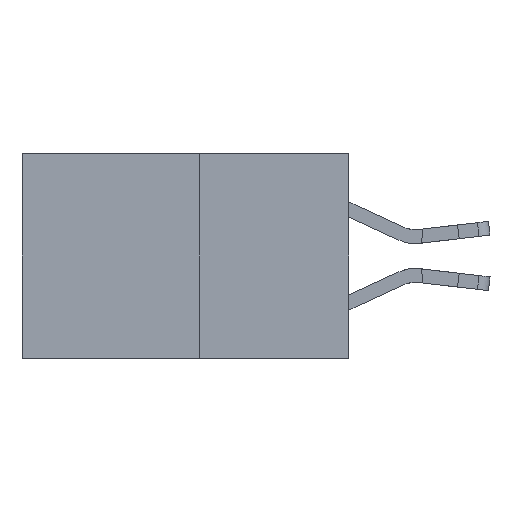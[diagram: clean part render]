
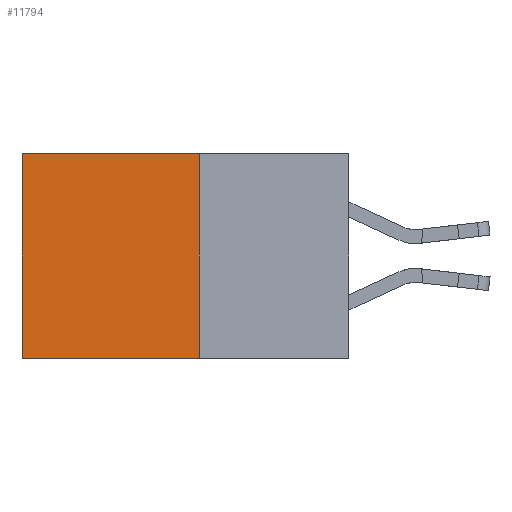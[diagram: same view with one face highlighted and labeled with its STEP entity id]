
A CAD part, left-side view. The second image highlights one B-rep face of the part: STEP entity #11794.
In plain terms, the highlighted planar face has unit normal (-1, 0, 0).
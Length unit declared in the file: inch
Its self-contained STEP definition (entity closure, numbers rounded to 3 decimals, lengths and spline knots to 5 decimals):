
#66 = LINE ( 'NONE', #465, #6955 ) ;
#70 = LINE ( 'NONE', #5146, #9962 ) ;
#465 = CARTESIAN_POINT ( 'NONE',  ( 0.277, 0.27, -0.37 ) ) ;
#1037 = CARTESIAN_POINT ( 'NONE',  ( 0.277, 0.59, -0.37 ) ) ;
#1251 = VERTEX_POINT ( 'NONE', #4423 ) ;
#1597 = EDGE_LOOP ( 'NONE', ( #9879, #11978, #2578, #4477 ) ) ;
#1881 = CARTESIAN_POINT ( 'NONE',  ( 0.277, 0.59, -0.37 ) ) ;
#2084 = FACE_OUTER_BOUND ( 'NONE', #1597, .T. ) ;
#2578 = ORIENTED_EDGE ( 'NONE', *, *, #8076, .F. ) ;
#3322 = DIRECTION ( 'NONE',  ( 0., 1., 0. ) ) ;
#3842 = CARTESIAN_POINT ( 'NONE',  ( 0.277, 0.27, -0.37 ) ) ;
#4030 = VECTOR ( 'NONE', #3322, 39.37008 ) ;
#4300 = DIRECTION ( 'NONE',  ( 0., 1., 0. ) ) ;
#4423 = CARTESIAN_POINT ( 'NONE',  ( 0.277, 0.27, 0. ) ) ;
#4427 = LINE ( 'NONE', #13517, #4030 ) ;
#4477 = ORIENTED_EDGE ( 'NONE', *, *, #15100, .T. ) ;
#5146 = CARTESIAN_POINT ( 'NONE',  ( 0.277, 0.27, -0.37 ) ) ;
#6451 = DIRECTION ( 'NONE',  ( 1., 0., 0. ) ) ;
#6955 = VECTOR ( 'NONE', #4300, 39.37008 ) ;
#6996 = VERTEX_POINT ( 'NONE', #1037 ) ;
#7364 = EDGE_CURVE ( 'NONE', #16278, #6996, #66, .T. ) ;
#7769 = AXIS2_PLACEMENT_3D ( 'NONE', #3842, #6451, #15382 ) ;
#8076 = EDGE_CURVE ( 'NONE', #1251, #16278, #70, .T. ) ;
#9434 = VERTEX_POINT ( 'NONE', #15636 ) ;
#9879 = ORIENTED_EDGE ( 'NONE', *, *, #12708, .T. ) ;
#9962 = VECTOR ( 'NONE', #12818, 39.37008 ) ;
#10826 = CARTESIAN_POINT ( 'NONE',  ( 0.277, 0.27, -0.37 ) ) ;
#11794 = ADVANCED_FACE ( 'NONE', ( #2084 ), #14094, .F. ) ;
#11901 = VECTOR ( 'NONE', #13457, 39.37008 ) ;
#11978 = ORIENTED_EDGE ( 'NONE', *, *, #7364, .F. ) ;
#12708 = EDGE_CURVE ( 'NONE', #9434, #6996, #15309, .T. ) ;
#12818 = DIRECTION ( 'NONE',  ( 0., 0., -1. ) ) ;
#13457 = DIRECTION ( 'NONE',  ( 0., 0., -1. ) ) ;
#13517 = CARTESIAN_POINT ( 'NONE',  ( 0.277, 0.27, 0. ) ) ;
#14094 = PLANE ( 'NONE',  #7769 ) ;
#15100 = EDGE_CURVE ( 'NONE', #1251, #9434, #4427, .T. ) ;
#15309 = LINE ( 'NONE', #1881, #11901 ) ;
#15382 = DIRECTION ( 'NONE',  ( 0., 0., -1. ) ) ;
#15636 = CARTESIAN_POINT ( 'NONE',  ( 0.277, 0.59, 0. ) ) ;
#16278 = VERTEX_POINT ( 'NONE', #10826 ) ;
